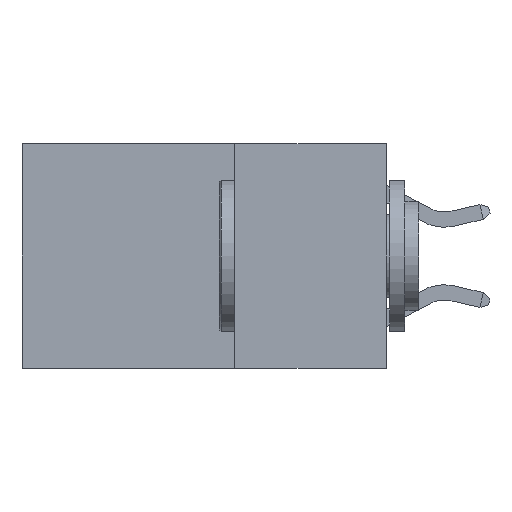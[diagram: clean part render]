
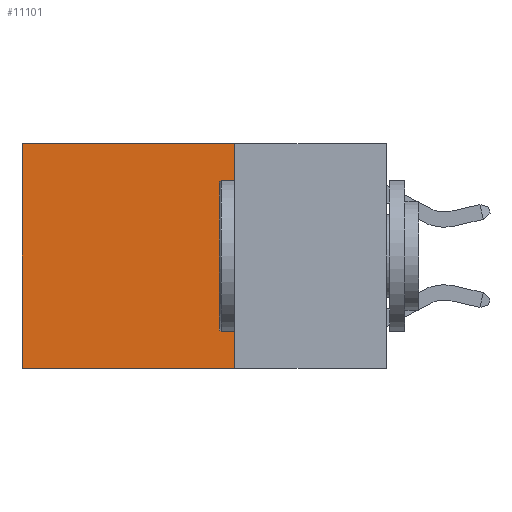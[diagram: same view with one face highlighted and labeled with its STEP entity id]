
A CAD part, left-side view. The second image highlights one B-rep face of the part: STEP entity #11101.
In plain terms, the highlighted planar face has unit normal (-1, 0, 0).
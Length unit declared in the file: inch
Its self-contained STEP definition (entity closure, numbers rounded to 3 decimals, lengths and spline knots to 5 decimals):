
#535 = EDGE_CURVE ( 'NONE', #8592, #6140, #7393, .T. ) ;
#793 = CARTESIAN_POINT ( 'NONE',  ( 0.2625, 0.25, -0.37 ) ) ;
#930 = CARTESIAN_POINT ( 'NONE',  ( 0.2625, 0.25, -0.37 ) ) ;
#2465 = CARTESIAN_POINT ( 'NONE',  ( 0.2625, 0.25, 0. ) ) ;
#2765 = DIRECTION ( 'NONE',  ( 0., 1., 0. ) ) ;
#3014 = DIRECTION ( 'NONE',  ( 1., 0., 0. ) ) ;
#3616 = DIRECTION ( 'NONE',  ( 0., 0., -1. ) ) ;
#3734 = EDGE_CURVE ( 'NONE', #6140, #4002, #4025, .T. ) ;
#3961 = PLANE ( 'NONE',  #11811 ) ;
#4002 = VERTEX_POINT ( 'NONE', #7751 ) ;
#4025 = LINE ( 'NONE', #793, #6891 ) ;
#4144 = VECTOR ( 'NONE', #2765, 39.37008 ) ;
#4262 = DIRECTION ( 'NONE',  ( 0., 0., -1. ) ) ;
#4457 = ORIENTED_EDGE ( 'NONE', *, *, #3734, .F. ) ;
#4747 = VECTOR ( 'NONE', #3616, 39.37008 ) ;
#5058 = EDGE_CURVE ( 'NONE', #8592, #5635, #6102, .T. ) ;
#5352 = LINE ( 'NONE', #11039, #4747 ) ;
#5635 = VERTEX_POINT ( 'NONE', #11476 ) ;
#6102 = LINE ( 'NONE', #9065, #4144 ) ;
#6140 = VERTEX_POINT ( 'NONE', #930 ) ;
#6891 = VECTOR ( 'NONE', #10427, 39.37008 ) ;
#7203 = EDGE_LOOP ( 'NONE', ( #9088, #4457, #11883, #9939 ) ) ;
#7393 = LINE ( 'NONE', #2465, #11777 ) ;
#7571 = CARTESIAN_POINT ( 'NONE',  ( 0.2625, 0.25, 0. ) ) ;
#7751 = CARTESIAN_POINT ( 'NONE',  ( 0.2625, 0.6, -0.37 ) ) ;
#8592 = VERTEX_POINT ( 'NONE', #7571 ) ;
#8742 = CARTESIAN_POINT ( 'NONE',  ( 0.2625, 0.25, 0. ) ) ;
#9065 = CARTESIAN_POINT ( 'NONE',  ( 0.2625, 0.25, 0. ) ) ;
#9088 = ORIENTED_EDGE ( 'NONE', *, *, #11397, .T. ) ;
#9939 = ORIENTED_EDGE ( 'NONE', *, *, #5058, .T. ) ;
#10427 = DIRECTION ( 'NONE',  ( 0., 1., 0. ) ) ;
#10516 = FACE_OUTER_BOUND ( 'NONE', #7203, .T. ) ;
#11039 = CARTESIAN_POINT ( 'NONE',  ( 0.2625, 0.6, 0. ) ) ;
#11101 = ADVANCED_FACE ( 'NONE', ( #10516 ), #3961, .F. ) ;
#11397 = EDGE_CURVE ( 'NONE', #5635, #4002, #5352, .T. ) ;
#11476 = CARTESIAN_POINT ( 'NONE',  ( 0.2625, 0.6, 0. ) ) ;
#11612 = DIRECTION ( 'NONE',  ( 0., 0., -1. ) ) ;
#11777 = VECTOR ( 'NONE', #4262, 39.37008 ) ;
#11811 = AXIS2_PLACEMENT_3D ( 'NONE', #8742, #3014, #11612 ) ;
#11883 = ORIENTED_EDGE ( 'NONE', *, *, #535, .F. ) ;
